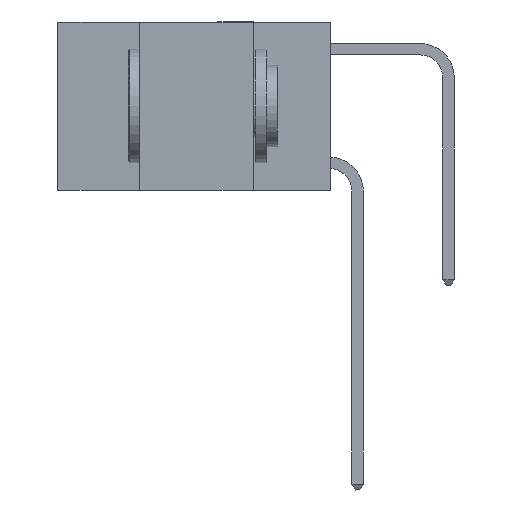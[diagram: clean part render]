
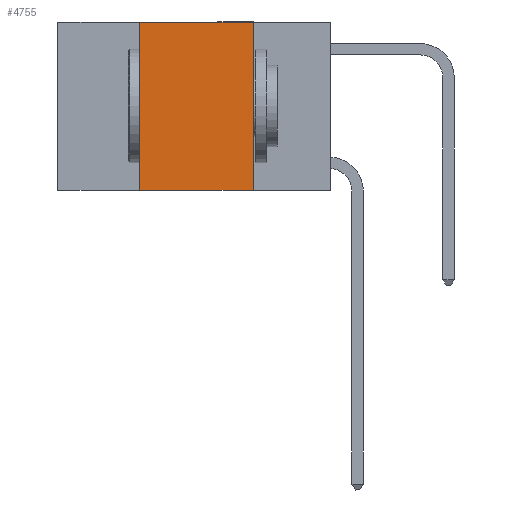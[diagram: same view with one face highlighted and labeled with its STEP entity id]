
A CAD part, left-side view. The second image highlights one B-rep face of the part: STEP entity #4755.
In plain terms, the highlighted planar face has unit normal (-1, 0, 0).
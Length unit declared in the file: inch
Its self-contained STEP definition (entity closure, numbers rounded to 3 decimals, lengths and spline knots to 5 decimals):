
#746 = CARTESIAN_POINT ( 'NONE',  ( 0., 0.42, -0.37 ) ) ;
#804 = VERTEX_POINT ( 'NONE', #2462 ) ;
#940 = DIRECTION ( 'NONE',  ( 0., 0., -1. ) ) ;
#1321 = EDGE_LOOP ( 'NONE', ( #10167, #7212, #9217, #8587 ) ) ;
#1490 = CARTESIAN_POINT ( 'NONE',  ( 0., 0.17, 0. ) ) ;
#1720 = FACE_OUTER_BOUND ( 'NONE', #1321, .T. ) ;
#1738 = DIRECTION ( 'NONE',  ( 0., 0., 1. ) ) ;
#2081 = VECTOR ( 'NONE', #7720, 39.37008 ) ;
#2462 = CARTESIAN_POINT ( 'NONE',  ( 0., 0.42, 0. ) ) ;
#2644 = LINE ( 'NONE', #3489, #6517 ) ;
#2759 = EDGE_CURVE ( 'NONE', #804, #3877, #2644, .T. ) ;
#3382 = VECTOR ( 'NONE', #1738, 39.37008 ) ;
#3386 = DIRECTION ( 'NONE',  ( 0., -1., 0. ) ) ;
#3448 = LINE ( 'NONE', #5955, #2081 ) ;
#3489 = CARTESIAN_POINT ( 'NONE',  ( 0., 0.6, 0. ) ) ;
#3877 = VERTEX_POINT ( 'NONE', #10952 ) ;
#4160 = LINE ( 'NONE', #1490, #9138 ) ;
#4336 = PLANE ( 'NONE',  #10957 ) ;
#4448 = CARTESIAN_POINT ( 'NONE',  ( 0., 0.6, 0. ) ) ;
#4731 = CARTESIAN_POINT ( 'NONE',  ( 0., 0.17, -0.37 ) ) ;
#4755 = ADVANCED_FACE ( 'NONE', ( #1720 ), #4336, .F. ) ;
#5955 = CARTESIAN_POINT ( 'NONE',  ( 0., 0.6, -0.37 ) ) ;
#5962 = EDGE_CURVE ( 'NONE', #10980, #9141, #3448, .T. ) ;
#6517 = VECTOR ( 'NONE', #3386, 39.37008 ) ;
#7212 = ORIENTED_EDGE ( 'NONE', *, *, #2759, .F. ) ;
#7509 = EDGE_CURVE ( 'NONE', #10980, #804, #10396, .T. ) ;
#7720 = DIRECTION ( 'NONE',  ( 0., -1., 0. ) ) ;
#8587 = ORIENTED_EDGE ( 'NONE', *, *, #5962, .T. ) ;
#9138 = VECTOR ( 'NONE', #9323, 39.37008 ) ;
#9141 = VERTEX_POINT ( 'NONE', #4731 ) ;
#9217 = ORIENTED_EDGE ( 'NONE', *, *, #7509, .F. ) ;
#9323 = DIRECTION ( 'NONE',  ( 0., 0., -1. ) ) ;
#9516 = CARTESIAN_POINT ( 'NONE',  ( 0., 0.42, 0. ) ) ;
#10167 = ORIENTED_EDGE ( 'NONE', *, *, #10937, .F. ) ;
#10396 = LINE ( 'NONE', #9516, #3382 ) ;
#10433 = DIRECTION ( 'NONE',  ( 1., 0., 0. ) ) ;
#10937 = EDGE_CURVE ( 'NONE', #3877, #9141, #4160, .T. ) ;
#10952 = CARTESIAN_POINT ( 'NONE',  ( 0., 0.17, 0. ) ) ;
#10957 = AXIS2_PLACEMENT_3D ( 'NONE', #4448, #10433, #940 ) ;
#10980 = VERTEX_POINT ( 'NONE', #746 ) ;
